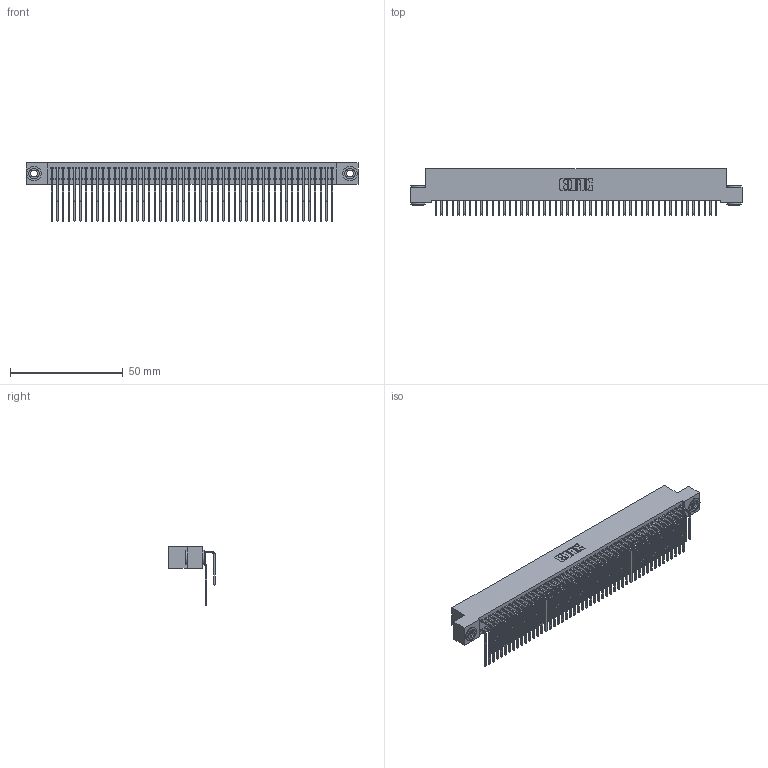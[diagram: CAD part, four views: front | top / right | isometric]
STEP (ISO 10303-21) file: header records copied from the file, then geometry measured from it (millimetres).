
FILE_DESCRIPTION (( 'STEP AP203' ), '1' );
FILE_NAME ('392-100-559-203.STEP', '2018-08-18T18:35:48', ( '' ), ( '' ), 'SwSTEP 2.0', 'SolidWorks 2016', '' );
FILE_SCHEMA (( 'CONFIG_CONTROL_DESIGN' ));
Length unit declared in the file: inch
Products named in the file (5): 342-250-002_345-250-002-102; 392-100-559-203; 342 Part_.156 TH; 345-292-001_558 559 Tail - 1; 345-292-001_559 Tail - 2
Assembly tree (103 placements, depth 2):
  392-100-559-203
    342 Part_.156 TH
    345-292-001_558 559 Tail - 1  x50
    345-292-001_559 Tail - 2  x50
    342-250-002_345-250-002-102  x2
Bounding box: 147.32 x 20.64 x 25.78 mm (x, y, z)
Volume: 13874.2 mm3; surface area: 25604.6 mm2
Topology: 103 solids, 103 shells, 5548 faces, 16475 edges, 10846 vertices
Faces by surface type: plane 3876, cylinder 1664, cone 8
Entity records: 33434 total; most frequent: CARTESIAN_POINT 5556, ORIENTED_EDGE 5434, DIRECTION 4747, EDGE_CURVE 2717, VECTOR 2525, LINE 2525, VERTEX_POINT 1806, AXIS2_PLACEMENT_3D 1111
